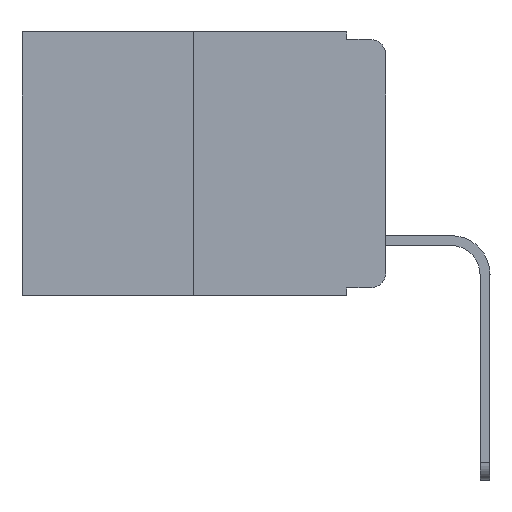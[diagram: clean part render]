
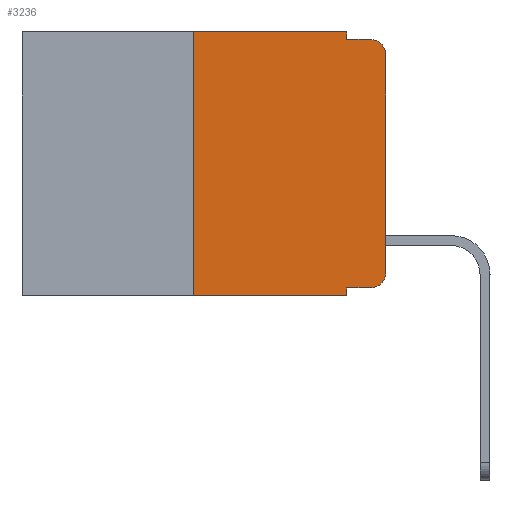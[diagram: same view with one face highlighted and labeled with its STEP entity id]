
A CAD part, left-side view. The second image highlights one B-rep face of the part: STEP entity #3236.
In plain terms, the highlighted planar face has unit normal (-1, 0, 0).
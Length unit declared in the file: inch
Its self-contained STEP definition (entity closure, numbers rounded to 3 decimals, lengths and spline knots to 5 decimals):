
#168 = DIRECTION ( 'NONE',  ( 0., 0., -1. ) ) ;
#604 = DIRECTION ( 'NONE',  ( 0., 0., -1. ) ) ;
#1078 = DIRECTION ( 'NONE',  ( 0., 0., -1. ) ) ;
#1401 = CARTESIAN_POINT ( 'NONE',  ( 0., 0.051, 0. ) ) ;
#1778 = VERTEX_POINT ( 'NONE', #1401 ) ;
#1817 = EDGE_CURVE ( 'NONE', #18648, #18584, #18784, .T. ) ;
#2037 = CARTESIAN_POINT ( 'NONE',  ( 0., 0.473, -0.343 ) ) ;
#2649 = DIRECTION ( 'NONE',  ( -1., 0., 0. ) ) ;
#3029 = ORIENTED_EDGE ( 'NONE', *, *, #13078, .T. ) ;
#3162 = VECTOR ( 'NONE', #4106, 39.37008 ) ;
#3206 = VERTEX_POINT ( 'NONE', #10935 ) ;
#3234 = LINE ( 'NONE', #20795, #7981 ) ;
#3236 = ADVANCED_FACE ( 'NONE', ( #14509 ), #12814, .F. ) ;
#3675 = EDGE_CURVE ( 'NONE', #1778, #18648, #11648, .T. ) ;
#3912 = DIRECTION ( 'NONE',  ( 1., 0., 0. ) ) ;
#4106 = DIRECTION ( 'NONE',  ( 0., 0., 1. ) ) ;
#4314 = EDGE_CURVE ( 'NONE', #3206, #21733, #23190, .T. ) ;
#4592 = ORIENTED_EDGE ( 'NONE', *, *, #15788, .T. ) ;
#4669 = CARTESIAN_POINT ( 'NONE',  ( 0., 0.051, 0. ) ) ;
#4757 = CARTESIAN_POINT ( 'NONE',  ( 0., 0.02, -0.03 ) ) ;
#4979 = EDGE_CURVE ( 'NONE', #9644, #15709, #15586, .T. ) ;
#5148 = VECTOR ( 'NONE', #604, 39.37008 ) ;
#5216 = CIRCLE ( 'NONE', #22490, 0.02 ) ;
#5412 = CARTESIAN_POINT ( 'NONE',  ( 0., 0.473, 0. ) ) ;
#5711 = ORIENTED_EDGE ( 'NONE', *, *, #1817, .F. ) ;
#5745 = CARTESIAN_POINT ( 'NONE',  ( 0., 0.25, 0. ) ) ;
#6506 = DIRECTION ( 'NONE',  ( 0., 0., 1. ) ) ;
#6582 = ORIENTED_EDGE ( 'NONE', *, *, #15434, .F. ) ;
#6844 = CARTESIAN_POINT ( 'NONE',  ( 0., 0., -0.03 ) ) ;
#7011 = VECTOR ( 'NONE', #10872, 39.37008 ) ;
#7529 = EDGE_CURVE ( 'NONE', #12304, #1778, #12233, .T. ) ;
#7632 = CARTESIAN_POINT ( 'NONE',  ( 0., 0.051, 0. ) ) ;
#7981 = VECTOR ( 'NONE', #20639, 39.37008 ) ;
#8454 = EDGE_LOOP ( 'NONE', ( #4592, #3029, #5711, #20867, #9674, #6582, #16983, #16667, #22388, #9710 ) ) ;
#9150 = DIRECTION ( 'NONE',  ( 0., -1., 0. ) ) ;
#9275 = LINE ( 'NONE', #2037, #7011 ) ;
#9568 = CARTESIAN_POINT ( 'NONE',  ( 0., 0.473, 0. ) ) ;
#9644 = VERTEX_POINT ( 'NONE', #15937 ) ;
#9674 = ORIENTED_EDGE ( 'NONE', *, *, #7529, .F. ) ;
#9710 = ORIENTED_EDGE ( 'NONE', *, *, #4979, .T. ) ;
#9732 = VERTEX_POINT ( 'NONE', #19202 ) ;
#10053 = DIRECTION ( 'NONE',  ( 0., 0., -1. ) ) ;
#10872 = DIRECTION ( 'NONE',  ( 0., -1., 0. ) ) ;
#10935 = CARTESIAN_POINT ( 'NONE',  ( 0., 0.051, -0.333 ) ) ;
#11445 = CARTESIAN_POINT ( 'NONE',  ( 0., 0.02, -0.01 ) ) ;
#11529 = CARTESIAN_POINT ( 'NONE',  ( 0., 0.25, 0. ) ) ;
#11593 = EDGE_CURVE ( 'NONE', #9732, #21733, #9275, .T. ) ;
#11648 = LINE ( 'NONE', #4669, #14489 ) ;
#12233 = LINE ( 'NONE', #9568, #17590 ) ;
#12304 = VERTEX_POINT ( 'NONE', #11529 ) ;
#12814 = PLANE ( 'NONE',  #18155 ) ;
#13078 = EDGE_CURVE ( 'NONE', #21820, #18584, #5216, .T. ) ;
#13533 = EDGE_CURVE ( 'NONE', #3206, #9644, #3234, .T. ) ;
#14130 = LINE ( 'NONE', #15456, #16373 ) ;
#14274 = AXIS2_PLACEMENT_3D ( 'NONE', #22396, #2649, #10053 ) ;
#14489 = VECTOR ( 'NONE', #19155, 39.37008 ) ;
#14509 = FACE_OUTER_BOUND ( 'NONE', #8454, .T. ) ;
#15037 = DIRECTION ( 'NONE',  ( 0., -1., 0. ) ) ;
#15434 = EDGE_CURVE ( 'NONE', #9732, #12304, #21477, .T. ) ;
#15456 = CARTESIAN_POINT ( 'NONE',  ( 0., 0., 0. ) ) ;
#15586 = CIRCLE ( 'NONE', #14274, 0.02 ) ;
#15709 = VERTEX_POINT ( 'NONE', #20868 ) ;
#15788 = EDGE_CURVE ( 'NONE', #15709, #21820, #14130, .T. ) ;
#15937 = CARTESIAN_POINT ( 'NONE',  ( 0., 0.02, -0.333 ) ) ;
#16373 = VECTOR ( 'NONE', #6506, 39.37008 ) ;
#16667 = ORIENTED_EDGE ( 'NONE', *, *, #4314, .F. ) ;
#16983 = ORIENTED_EDGE ( 'NONE', *, *, #11593, .T. ) ;
#17590 = VECTOR ( 'NONE', #15037, 39.37008 ) ;
#18155 = AXIS2_PLACEMENT_3D ( 'NONE', #5412, #3912, #168 ) ;
#18410 = CARTESIAN_POINT ( 'NONE',  ( 0., 0.051, -0.343 ) ) ;
#18456 = CARTESIAN_POINT ( 'NONE',  ( 0., 0.051, -0.01 ) ) ;
#18584 = VERTEX_POINT ( 'NONE', #11445 ) ;
#18648 = VERTEX_POINT ( 'NONE', #18456 ) ;
#18784 = LINE ( 'NONE', #23198, #20748 ) ;
#19155 = DIRECTION ( 'NONE',  ( 0., 0., -1. ) ) ;
#19202 = CARTESIAN_POINT ( 'NONE',  ( 0., 0.25, -0.343 ) ) ;
#20639 = DIRECTION ( 'NONE',  ( 0., -1., 0. ) ) ;
#20748 = VECTOR ( 'NONE', #9150, 39.37008 ) ;
#20795 = CARTESIAN_POINT ( 'NONE',  ( 0., 0.051, -0.333 ) ) ;
#20867 = ORIENTED_EDGE ( 'NONE', *, *, #3675, .F. ) ;
#20868 = CARTESIAN_POINT ( 'NONE',  ( 0., 0., -0.313 ) ) ;
#21477 = LINE ( 'NONE', #5745, #3162 ) ;
#21733 = VERTEX_POINT ( 'NONE', #18410 ) ;
#21820 = VERTEX_POINT ( 'NONE', #6844 ) ;
#22388 = ORIENTED_EDGE ( 'NONE', *, *, #13533, .T. ) ;
#22396 = CARTESIAN_POINT ( 'NONE',  ( 0., 0.02, -0.313 ) ) ;
#22490 = AXIS2_PLACEMENT_3D ( 'NONE', #4757, #23273, #1078 ) ;
#23190 = LINE ( 'NONE', #7632, #5148 ) ;
#23198 = CARTESIAN_POINT ( 'NONE',  ( 0., 0.051, -0.01 ) ) ;
#23273 = DIRECTION ( 'NONE',  ( -1., 0., 0. ) ) ;
